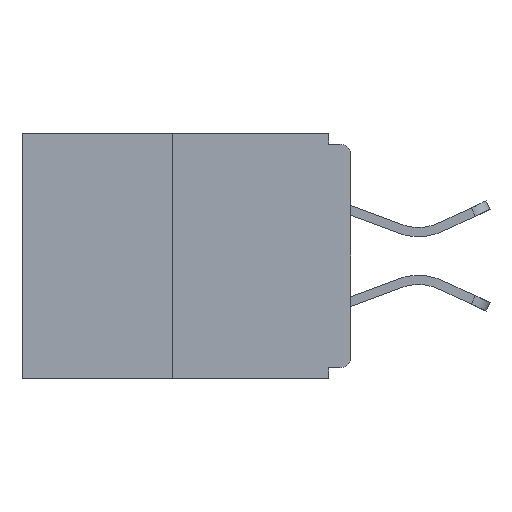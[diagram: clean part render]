
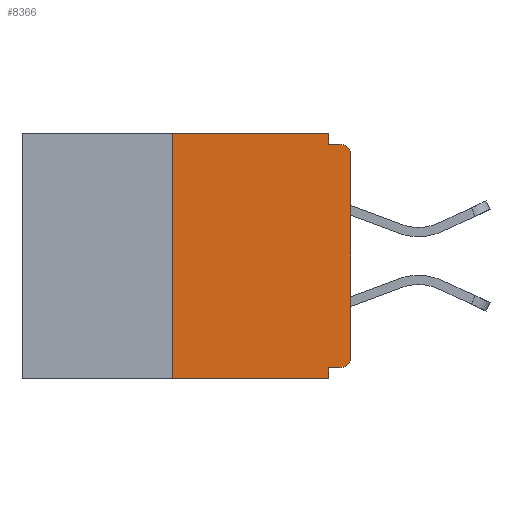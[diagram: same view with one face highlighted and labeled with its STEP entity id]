
A CAD part, left-side view. The second image highlights one B-rep face of the part: STEP entity #8366.
In plain terms, the highlighted planar face has unit normal (-1, 0, 0).
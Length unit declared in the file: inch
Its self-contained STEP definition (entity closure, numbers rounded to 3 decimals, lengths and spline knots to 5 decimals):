
#88 = EDGE_CURVE ( 'NONE', #8170, #13721, #21155, .T. ) ;
#441 = CARTESIAN_POINT ( 'NONE',  ( 0., 0.031, -0.328 ) ) ;
#554 = EDGE_CURVE ( 'NONE', #18378, #16378, #29308, .T. ) ;
#754 = LINE ( 'NONE', #3114, #7101 ) ;
#885 = ORIENTED_EDGE ( 'NONE', *, *, #23598, .F. ) ;
#1693 = AXIS2_PLACEMENT_3D ( 'NONE', #4725, #20581, #6999 ) ;
#1898 = EDGE_CURVE ( 'NONE', #8170, #4955, #17526, .T. ) ;
#1980 = CARTESIAN_POINT ( 'NONE',  ( 0., 0., -0.328 ) ) ;
#2438 = AXIS2_PLACEMENT_3D ( 'NONE', #4951, #5237, #14460 ) ;
#2797 = EDGE_CURVE ( 'NONE', #4955, #9861, #22097, .T. ) ;
#2835 = CARTESIAN_POINT ( 'NONE',  ( 0., 0.25, 0. ) ) ;
#3114 = CARTESIAN_POINT ( 'NONE',  ( 0., 0.46, -0.343 ) ) ;
#3142 = LINE ( 'NONE', #19362, #10600 ) ;
#3207 = VECTOR ( 'NONE', #12979, 39.37008 ) ;
#3358 = CARTESIAN_POINT ( 'NONE',  ( 0., 0., -0.313 ) ) ;
#3490 = ORIENTED_EDGE ( 'NONE', *, *, #12738, .T. ) ;
#4207 = PLANE ( 'NONE',  #25755 ) ;
#4725 = CARTESIAN_POINT ( 'NONE',  ( 0., 0.015, -0.03 ) ) ;
#4951 = CARTESIAN_POINT ( 'NONE',  ( 0., 0.015, -0.313 ) ) ;
#4955 = VERTEX_POINT ( 'NONE', #441 ) ;
#5237 = DIRECTION ( 'NONE',  ( -1., 0., 0. ) ) ;
#6006 = ORIENTED_EDGE ( 'NONE', *, *, #22266, .T. ) ;
#6279 = LINE ( 'NONE', #2835, #6979 ) ;
#6868 = EDGE_CURVE ( 'NONE', #25058, #16378, #3142, .T. ) ;
#6979 = VECTOR ( 'NONE', #14202, 39.37008 ) ;
#6999 = DIRECTION ( 'NONE',  ( 0., 0., -1. ) ) ;
#7101 = VECTOR ( 'NONE', #7373, 39.37008 ) ;
#7373 = DIRECTION ( 'NONE',  ( 0., -1., 0. ) ) ;
#8056 = ORIENTED_EDGE ( 'NONE', *, *, #88, .T. ) ;
#8094 = LINE ( 'NONE', #12540, #18005 ) ;
#8112 = ORIENTED_EDGE ( 'NONE', *, *, #23091, .F. ) ;
#8170 = VERTEX_POINT ( 'NONE', #10380 ) ;
#8366 = ADVANCED_FACE ( 'NONE', ( #23632 ), #4207, .F. ) ;
#9202 = ORIENTED_EDGE ( 'NONE', *, *, #554, .T. ) ;
#9543 = VERTEX_POINT ( 'NONE', #21168 ) ;
#9861 = VERTEX_POINT ( 'NONE', #13033 ) ;
#10171 = DIRECTION ( 'NONE',  ( 0., -1., 0. ) ) ;
#10380 = CARTESIAN_POINT ( 'NONE',  ( 0., 0.015, -0.328 ) ) ;
#10600 = VECTOR ( 'NONE', #10171, 39.37008 ) ;
#10936 = CARTESIAN_POINT ( 'NONE',  ( 0., 0.46, 0. ) ) ;
#11389 = LINE ( 'NONE', #10936, #3207 ) ;
#11895 = DIRECTION ( 'NONE',  ( 0., 0., -1. ) ) ;
#12540 = CARTESIAN_POINT ( 'NONE',  ( 0., 0., 0. ) ) ;
#12738 = EDGE_CURVE ( 'NONE', #13856, #9861, #754, .T. ) ;
#12979 = DIRECTION ( 'NONE',  ( 0., -1., 0. ) ) ;
#12990 = CARTESIAN_POINT ( 'NONE',  ( 0., 0.031, 0. ) ) ;
#13033 = CARTESIAN_POINT ( 'NONE',  ( 0., 0.031, -0.343 ) ) ;
#13211 = DIRECTION ( 'NONE',  ( 0., 0., -1. ) ) ;
#13419 = CARTESIAN_POINT ( 'NONE',  ( 0., 0., -0.03 ) ) ;
#13583 = CARTESIAN_POINT ( 'NONE',  ( 0., 0.031, -0.015 ) ) ;
#13721 = VERTEX_POINT ( 'NONE', #3358 ) ;
#13856 = VERTEX_POINT ( 'NONE', #26635 ) ;
#14202 = DIRECTION ( 'NONE',  ( 0., 0., 1. ) ) ;
#14460 = DIRECTION ( 'NONE',  ( 0., 0., -1. ) ) ;
#14888 = VERTEX_POINT ( 'NONE', #29270 ) ;
#15289 = EDGE_CURVE ( 'NONE', #9543, #14888, #11389, .T. ) ;
#16378 = VERTEX_POINT ( 'NONE', #21832 ) ;
#16826 = VECTOR ( 'NONE', #26826, 39.37008 ) ;
#17051 = EDGE_LOOP ( 'NONE', ( #27534, #8112, #3490, #26142, #20185, #8056, #6006, #9202, #23576, #885 ) ) ;
#17526 = LINE ( 'NONE', #1980, #16826 ) ;
#18005 = VECTOR ( 'NONE', #28465, 39.37008 ) ;
#18378 = VERTEX_POINT ( 'NONE', #13419 ) ;
#18646 = VECTOR ( 'NONE', #22105, 39.37008 ) ;
#18904 = CARTESIAN_POINT ( 'NONE',  ( 0., 0.031, -0.343 ) ) ;
#19362 = CARTESIAN_POINT ( 'NONE',  ( 0., 0., -0.015 ) ) ;
#20185 = ORIENTED_EDGE ( 'NONE', *, *, #1898, .F. ) ;
#20581 = DIRECTION ( 'NONE',  ( -1., 0., 0. ) ) ;
#21155 = CIRCLE ( 'NONE', #2438, 0.015 ) ;
#21168 = CARTESIAN_POINT ( 'NONE',  ( 0., 0.25, 0. ) ) ;
#21832 = CARTESIAN_POINT ( 'NONE',  ( 0., 0.015, -0.015 ) ) ;
#22097 = LINE ( 'NONE', #18904, #23913 ) ;
#22105 = DIRECTION ( 'NONE',  ( 0., 0., -1. ) ) ;
#22266 = EDGE_CURVE ( 'NONE', #13721, #18378, #8094, .T. ) ;
#22320 = DIRECTION ( 'NONE',  ( 1., 0., 0. ) ) ;
#23091 = EDGE_CURVE ( 'NONE', #13856, #9543, #6279, .T. ) ;
#23576 = ORIENTED_EDGE ( 'NONE', *, *, #6868, .F. ) ;
#23598 = EDGE_CURVE ( 'NONE', #14888, #25058, #28922, .T. ) ;
#23632 = FACE_OUTER_BOUND ( 'NONE', #17051, .T. ) ;
#23913 = VECTOR ( 'NONE', #11895, 39.37008 ) ;
#25058 = VERTEX_POINT ( 'NONE', #13583 ) ;
#25755 = AXIS2_PLACEMENT_3D ( 'NONE', #29368, #22320, #13211 ) ;
#26142 = ORIENTED_EDGE ( 'NONE', *, *, #2797, .F. ) ;
#26635 = CARTESIAN_POINT ( 'NONE',  ( 0., 0.25, -0.343 ) ) ;
#26826 = DIRECTION ( 'NONE',  ( 0., 1., 0. ) ) ;
#27534 = ORIENTED_EDGE ( 'NONE', *, *, #15289, .F. ) ;
#28465 = DIRECTION ( 'NONE',  ( 0., 0., 1. ) ) ;
#28922 = LINE ( 'NONE', #12990, #18646 ) ;
#29270 = CARTESIAN_POINT ( 'NONE',  ( 0., 0.031, 0. ) ) ;
#29308 = CIRCLE ( 'NONE', #1693, 0.015 ) ;
#29368 = CARTESIAN_POINT ( 'NONE',  ( 0., 0.46, 0. ) ) ;
